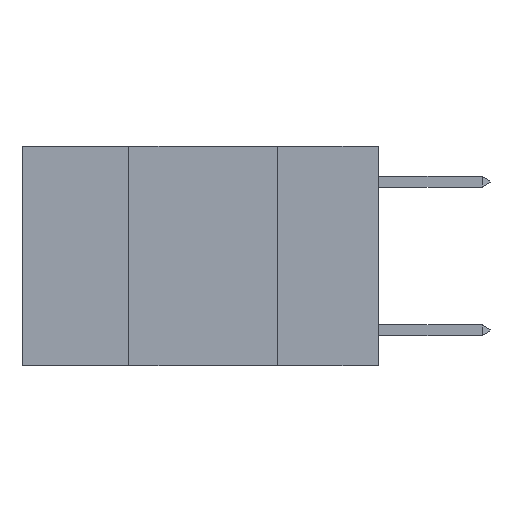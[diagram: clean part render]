
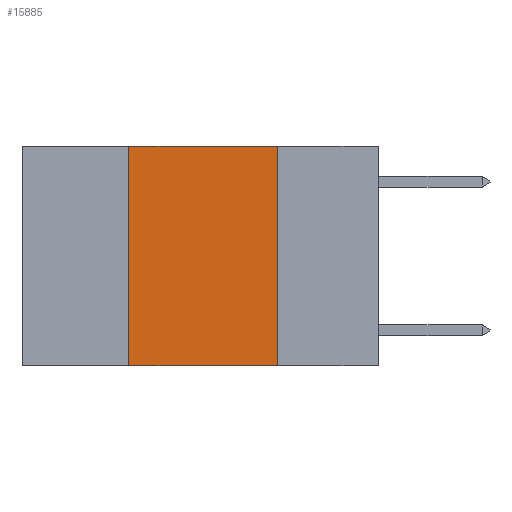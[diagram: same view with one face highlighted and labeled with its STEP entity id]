
A CAD part, left-side view. The second image highlights one B-rep face of the part: STEP entity #15885.
In plain terms, the highlighted planar face has unit normal (-1, 0, 0).
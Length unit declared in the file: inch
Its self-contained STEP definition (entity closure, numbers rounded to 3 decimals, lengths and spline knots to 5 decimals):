
#1252 = DIRECTION ( 'NONE',  ( 0., -1., 0. ) ) ;
#2805 = EDGE_CURVE ( 'NONE', #8522, #12645, #8617, .T. ) ;
#2861 = EDGE_LOOP ( 'NONE', ( #5194, #5295, #5729, #5750 ) ) ;
#3119 = LINE ( 'NONE', #11498, #12131 ) ;
#3530 = CARTESIAN_POINT ( 'NONE',  ( 0., 0.42, 0. ) ) ;
#3947 = EDGE_CURVE ( 'NONE', #8522, #7667, #17610, .T. ) ;
#4162 = DIRECTION ( 'NONE',  ( 0., -1., 0. ) ) ;
#4263 = CARTESIAN_POINT ( 'NONE',  ( 0., 0.6, -0.37 ) ) ;
#5105 = EDGE_CURVE ( 'NONE', #7300, #12645, #19819, .T. ) ;
#5194 = ORIENTED_EDGE ( 'NONE', *, *, #5105, .F. ) ;
#5295 = ORIENTED_EDGE ( 'NONE', *, *, #12486, .F. ) ;
#5729 = ORIENTED_EDGE ( 'NONE', *, *, #3947, .F. ) ;
#5750 = ORIENTED_EDGE ( 'NONE', *, *, #2805, .T. ) ;
#6142 = DIRECTION ( 'NONE',  ( 0., 0., -1. ) ) ;
#6573 = DIRECTION ( 'NONE',  ( 0., 0., 1. ) ) ;
#6723 = CARTESIAN_POINT ( 'NONE',  ( 0., 0.42, 0. ) ) ;
#7073 = FACE_OUTER_BOUND ( 'NONE', #2861, .T. ) ;
#7300 = VERTEX_POINT ( 'NONE', #14285 ) ;
#7667 = VERTEX_POINT ( 'NONE', #3530 ) ;
#7774 = CARTESIAN_POINT ( 'NONE',  ( 0., 0.6, 0. ) ) ;
#8522 = VERTEX_POINT ( 'NONE', #10981 ) ;
#8617 = LINE ( 'NONE', #4263, #12583 ) ;
#10981 = CARTESIAN_POINT ( 'NONE',  ( 0., 0.42, -0.37 ) ) ;
#11498 = CARTESIAN_POINT ( 'NONE',  ( 0., 0.6, 0. ) ) ;
#12131 = VECTOR ( 'NONE', #1252, 39.37008 ) ;
#12486 = EDGE_CURVE ( 'NONE', #7667, #7300, #3119, .T. ) ;
#12583 = VECTOR ( 'NONE', #4162, 39.37008 ) ;
#12645 = VERTEX_POINT ( 'NONE', #13751 ) ;
#13308 = VECTOR ( 'NONE', #6573, 39.37008 ) ;
#13751 = CARTESIAN_POINT ( 'NONE',  ( 0., 0.17, -0.37 ) ) ;
#14285 = CARTESIAN_POINT ( 'NONE',  ( 0., 0.17, 0. ) ) ;
#15885 = ADVANCED_FACE ( 'NONE', ( #7073 ), #17692, .F. ) ;
#16080 = VECTOR ( 'NONE', #17347, 39.37008 ) ;
#16170 = DIRECTION ( 'NONE',  ( 1., 0., 0. ) ) ;
#17347 = DIRECTION ( 'NONE',  ( 0., 0., -1. ) ) ;
#17397 = CARTESIAN_POINT ( 'NONE',  ( 0., 0.17, 0. ) ) ;
#17610 = LINE ( 'NONE', #6723, #13308 ) ;
#17692 = PLANE ( 'NONE',  #20755 ) ;
#19819 = LINE ( 'NONE', #17397, #16080 ) ;
#20755 = AXIS2_PLACEMENT_3D ( 'NONE', #7774, #16170, #6142 ) ;
